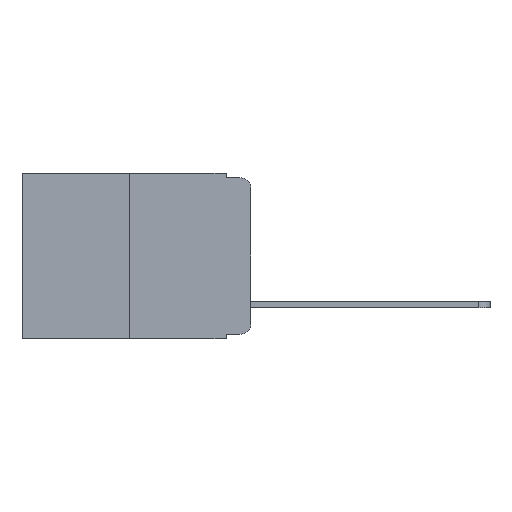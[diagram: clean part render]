
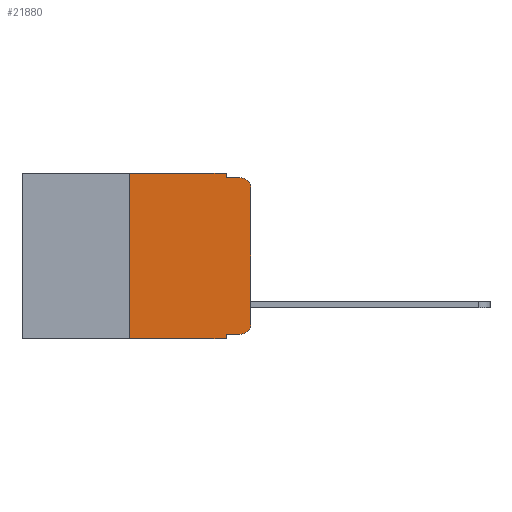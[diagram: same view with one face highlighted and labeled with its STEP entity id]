
A CAD part, left-side view. The second image highlights one B-rep face of the part: STEP entity #21880.
In plain terms, the highlighted planar face has unit normal (-1, 0, 0).
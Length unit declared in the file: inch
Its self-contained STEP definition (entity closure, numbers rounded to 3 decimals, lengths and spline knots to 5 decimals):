
#72 = ORIENTED_EDGE ( 'NONE', *, *, #11412, .T. ) ;
#260 = VERTEX_POINT ( 'NONE', #22266 ) ;
#360 = CARTESIAN_POINT ( 'NONE',  ( 0., 0.051, 0. ) ) ;
#463 = LINE ( 'NONE', #8577, #20623 ) ;
#485 = VERTEX_POINT ( 'NONE', #14681 ) ;
#733 = ORIENTED_EDGE ( 'NONE', *, *, #19496, .T. ) ;
#1172 = ORIENTED_EDGE ( 'NONE', *, *, #23722, .F. ) ;
#1294 = VECTOR ( 'NONE', #23579, 39.37008 ) ;
#1443 = VECTOR ( 'NONE', #17164, 39.37008 ) ;
#1639 = EDGE_CURVE ( 'NONE', #13422, #17506, #463, .T. ) ;
#2848 = VERTEX_POINT ( 'NONE', #21587 ) ;
#2854 = DIRECTION ( 'NONE',  ( 0., -1., 0. ) ) ;
#3746 = CARTESIAN_POINT ( 'NONE',  ( 0., 0.051, -0.01 ) ) ;
#4335 = ORIENTED_EDGE ( 'NONE', *, *, #1639, .F. ) ;
#4436 = VERTEX_POINT ( 'NONE', #15876 ) ;
#4989 = EDGE_CURVE ( 'NONE', #485, #8448, #15893, .T. ) ;
#5170 = AXIS2_PLACEMENT_3D ( 'NONE', #22515, #24408, #13470 ) ;
#5476 = CARTESIAN_POINT ( 'NONE',  ( 0., 0.02, -0.03 ) ) ;
#5791 = EDGE_CURVE ( 'NONE', #4436, #260, #8006, .T. ) ;
#5797 = DIRECTION ( 'NONE',  ( 0., -1., 0. ) ) ;
#6317 = CARTESIAN_POINT ( 'NONE',  ( 0., 0.02, -0.313 ) ) ;
#6479 = VERTEX_POINT ( 'NONE', #18211 ) ;
#6545 = ORIENTED_EDGE ( 'NONE', *, *, #5791, .F. ) ;
#6550 = DIRECTION ( 'NONE',  ( 0., -1., 0. ) ) ;
#7370 = VECTOR ( 'NONE', #21426, 39.37008 ) ;
#7502 = DIRECTION ( 'NONE',  ( 0., 0., -1. ) ) ;
#7799 = ORIENTED_EDGE ( 'NONE', *, *, #11656, .T. ) ;
#8006 = LINE ( 'NONE', #10302, #7370 ) ;
#8222 = VECTOR ( 'NONE', #2854, 39.37008 ) ;
#8373 = DIRECTION ( 'NONE',  ( 0., 0., -1. ) ) ;
#8448 = VERTEX_POINT ( 'NONE', #22913 ) ;
#8577 = CARTESIAN_POINT ( 'NONE',  ( 0., 0.473, 0. ) ) ;
#8975 = CARTESIAN_POINT ( 'NONE',  ( 0., 0.051, -0.333 ) ) ;
#9383 = EDGE_CURVE ( 'NONE', #14068, #13422, #12701, .T. ) ;
#9591 = PLANE ( 'NONE',  #5170 ) ;
#10302 = CARTESIAN_POINT ( 'NONE',  ( 0., 0.051, 0. ) ) ;
#10331 = CARTESIAN_POINT ( 'NONE',  ( 0., 0.25, -0.343 ) ) ;
#10819 = VECTOR ( 'NONE', #11119, 39.37008 ) ;
#10898 = VECTOR ( 'NONE', #5797, 39.37008 ) ;
#11119 = DIRECTION ( 'NONE',  ( 0., -1., 0. ) ) ;
#11192 = CARTESIAN_POINT ( 'NONE',  ( 0., 0.051, 0. ) ) ;
#11412 = EDGE_CURVE ( 'NONE', #14068, #260, #15822, .T. ) ;
#11646 = LINE ( 'NONE', #20780, #1443 ) ;
#11656 = EDGE_CURVE ( 'NONE', #2848, #6479, #20425, .T. ) ;
#12701 = LINE ( 'NONE', #20045, #1294 ) ;
#12772 = ORIENTED_EDGE ( 'NONE', *, *, #19536, .T. ) ;
#12994 = CARTESIAN_POINT ( 'NONE',  ( 0., 0., -0.03 ) ) ;
#13422 = VERTEX_POINT ( 'NONE', #21260 ) ;
#13470 = DIRECTION ( 'NONE',  ( 0., 0., -1. ) ) ;
#14068 = VERTEX_POINT ( 'NONE', #10331 ) ;
#14246 = ORIENTED_EDGE ( 'NONE', *, *, #9383, .F. ) ;
#14681 = CARTESIAN_POINT ( 'NONE',  ( 0., 0.051, -0.01 ) ) ;
#14825 = CARTESIAN_POINT ( 'NONE',  ( 0., 0.473, -0.343 ) ) ;
#14891 = VERTEX_POINT ( 'NONE', #12994 ) ;
#15822 = LINE ( 'NONE', #14825, #10819 ) ;
#15876 = CARTESIAN_POINT ( 'NONE',  ( 0., 0.051, -0.333 ) ) ;
#15893 = LINE ( 'NONE', #3746, #10898 ) ;
#16509 = EDGE_CURVE ( 'NONE', #4436, #2848, #19488, .T. ) ;
#17164 = DIRECTION ( 'NONE',  ( 0., 0., 1. ) ) ;
#17506 = VERTEX_POINT ( 'NONE', #360 ) ;
#17956 = LINE ( 'NONE', #11192, #22229 ) ;
#18211 = CARTESIAN_POINT ( 'NONE',  ( 0., 0., -0.313 ) ) ;
#18598 = DIRECTION ( 'NONE',  ( 0., 0., -1. ) ) ;
#18677 = EDGE_LOOP ( 'NONE', ( #12772, #733, #23085, #1172, #4335, #14246, #72, #6545, #20001, #7799 ) ) ;
#18943 = DIRECTION ( 'NONE',  ( -1., 0., 0. ) ) ;
#19488 = LINE ( 'NONE', #8975, #8222 ) ;
#19496 = EDGE_CURVE ( 'NONE', #14891, #8448, #22037, .T. ) ;
#19536 = EDGE_CURVE ( 'NONE', #6479, #14891, #11646, .T. ) ;
#19714 = DIRECTION ( 'NONE',  ( -1., 0., 0. ) ) ;
#19776 = AXIS2_PLACEMENT_3D ( 'NONE', #5476, #18943, #7502 ) ;
#19945 = AXIS2_PLACEMENT_3D ( 'NONE', #6317, #19714, #8373 ) ;
#20001 = ORIENTED_EDGE ( 'NONE', *, *, #16509, .T. ) ;
#20045 = CARTESIAN_POINT ( 'NONE',  ( 0., 0.25, 0. ) ) ;
#20425 = CIRCLE ( 'NONE', #19945, 0.02 ) ;
#20623 = VECTOR ( 'NONE', #6550, 39.37008 ) ;
#20780 = CARTESIAN_POINT ( 'NONE',  ( 0., 0., 0. ) ) ;
#21260 = CARTESIAN_POINT ( 'NONE',  ( 0., 0.25, 0. ) ) ;
#21426 = DIRECTION ( 'NONE',  ( 0., 0., -1. ) ) ;
#21587 = CARTESIAN_POINT ( 'NONE',  ( 0., 0.02, -0.333 ) ) ;
#21880 = ADVANCED_FACE ( 'NONE', ( #23989 ), #9591, .F. ) ;
#22037 = CIRCLE ( 'NONE', #19776, 0.02 ) ;
#22229 = VECTOR ( 'NONE', #18598, 39.37008 ) ;
#22266 = CARTESIAN_POINT ( 'NONE',  ( 0., 0.051, -0.343 ) ) ;
#22515 = CARTESIAN_POINT ( 'NONE',  ( 0., 0.473, 0. ) ) ;
#22913 = CARTESIAN_POINT ( 'NONE',  ( 0., 0.02, -0.01 ) ) ;
#23085 = ORIENTED_EDGE ( 'NONE', *, *, #4989, .F. ) ;
#23579 = DIRECTION ( 'NONE',  ( 0., 0., 1. ) ) ;
#23722 = EDGE_CURVE ( 'NONE', #17506, #485, #17956, .T. ) ;
#23989 = FACE_OUTER_BOUND ( 'NONE', #18677, .T. ) ;
#24408 = DIRECTION ( 'NONE',  ( 1., 0., 0. ) ) ;
